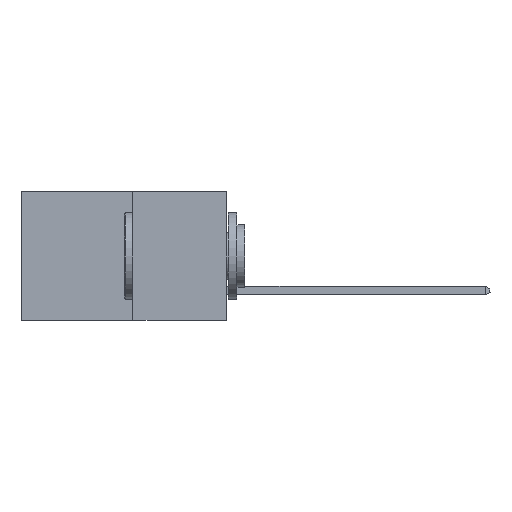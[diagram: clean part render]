
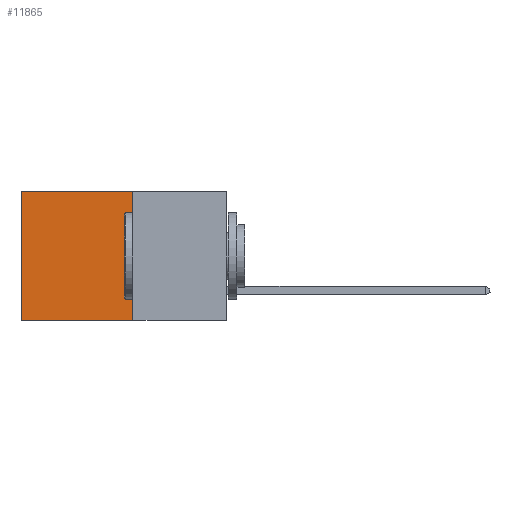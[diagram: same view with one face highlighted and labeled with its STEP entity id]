
A CAD part, left-side view. The second image highlights one B-rep face of the part: STEP entity #11865.
In plain terms, the highlighted planar face has unit normal (-1, 0, 0).
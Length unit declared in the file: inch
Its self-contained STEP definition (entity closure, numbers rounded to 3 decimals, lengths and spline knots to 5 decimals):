
#1285 = VECTOR ( 'NONE', #17378, 39.37008 ) ;
#1824 = EDGE_CURVE ( 'NONE', #10687, #16219, #12517, .T. ) ;
#2066 = DIRECTION ( 'NONE',  ( 0., 1., 0. ) ) ;
#2068 = VERTEX_POINT ( 'NONE', #8967 ) ;
#2203 = ORIENTED_EDGE ( 'NONE', *, *, #1824, .T. ) ;
#2224 = FACE_OUTER_BOUND ( 'NONE', #10888, .T. ) ;
#2310 = DIRECTION ( 'NONE',  ( 1., 0., 0. ) ) ;
#4622 = AXIS2_PLACEMENT_3D ( 'NONE', #10841, #2310, #12261 ) ;
#4989 = CARTESIAN_POINT ( 'NONE',  ( 0.277, 0.27, 0. ) ) ;
#5619 = ORIENTED_EDGE ( 'NONE', *, *, #7341, .F. ) ;
#5625 = CARTESIAN_POINT ( 'NONE',  ( 0.277, 0.59, 0. ) ) ;
#6062 = LINE ( 'NONE', #16017, #1285 ) ;
#6309 = CARTESIAN_POINT ( 'NONE',  ( 0.277, 0.59, -0.37 ) ) ;
#6915 = EDGE_CURVE ( 'NONE', #10784, #2068, #12243, .T. ) ;
#7341 = EDGE_CURVE ( 'NONE', #2068, #16219, #6062, .T. ) ;
#8029 = PLANE ( 'NONE',  #4622 ) ;
#8103 = EDGE_CURVE ( 'NONE', #10784, #10687, #17841, .T. ) ;
#8967 = CARTESIAN_POINT ( 'NONE',  ( 0.277, 0.27, -0.37 ) ) ;
#10687 = VERTEX_POINT ( 'NONE', #5625 ) ;
#10784 = VERTEX_POINT ( 'NONE', #12833 ) ;
#10841 = CARTESIAN_POINT ( 'NONE',  ( 0.277, 0.27, -0.37 ) ) ;
#10888 = EDGE_LOOP ( 'NONE', ( #2203, #5619, #14133, #10993 ) ) ;
#10993 = ORIENTED_EDGE ( 'NONE', *, *, #8103, .T. ) ;
#11865 = ADVANCED_FACE ( 'NONE', ( #2224 ), #8029, .F. ) ;
#12195 = CARTESIAN_POINT ( 'NONE',  ( 0.277, 0.27, -0.37 ) ) ;
#12243 = LINE ( 'NONE', #12195, #15520 ) ;
#12261 = DIRECTION ( 'NONE',  ( 0., 0., -1. ) ) ;
#12517 = LINE ( 'NONE', #14066, #15363 ) ;
#12833 = CARTESIAN_POINT ( 'NONE',  ( 0.277, 0.27, 0. ) ) ;
#14066 = CARTESIAN_POINT ( 'NONE',  ( 0.277, 0.59, -0.37 ) ) ;
#14133 = ORIENTED_EDGE ( 'NONE', *, *, #6915, .F. ) ;
#14487 = DIRECTION ( 'NONE',  ( 0., 0., -1. ) ) ;
#15363 = VECTOR ( 'NONE', #14487, 39.37008 ) ;
#15520 = VECTOR ( 'NONE', #16423, 39.37008 ) ;
#16017 = CARTESIAN_POINT ( 'NONE',  ( 0.277, 0.27, -0.37 ) ) ;
#16219 = VERTEX_POINT ( 'NONE', #6309 ) ;
#16423 = DIRECTION ( 'NONE',  ( 0., 0., -1. ) ) ;
#17378 = DIRECTION ( 'NONE',  ( 0., 1., 0. ) ) ;
#17420 = VECTOR ( 'NONE', #2066, 39.37008 ) ;
#17841 = LINE ( 'NONE', #4989, #17420 ) ;
